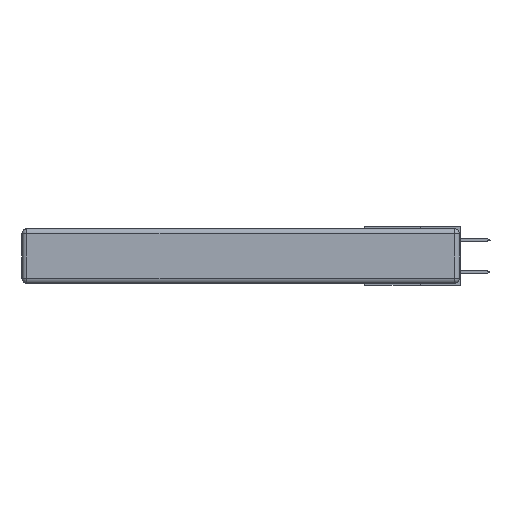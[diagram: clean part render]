
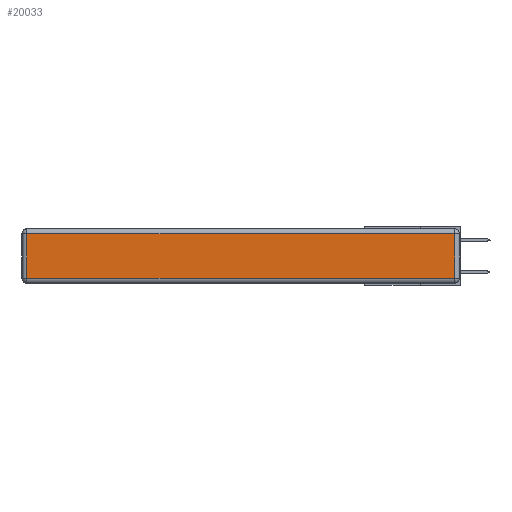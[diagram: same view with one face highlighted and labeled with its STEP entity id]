
A CAD part, left-side view. The second image highlights one B-rep face of the part: STEP entity #20033.
In plain terms, the highlighted planar face has unit normal (-1, 0, 0).
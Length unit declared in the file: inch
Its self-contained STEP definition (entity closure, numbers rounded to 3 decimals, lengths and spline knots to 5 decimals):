
#385 = DIRECTION ( 'NONE',  ( 0., 0., 1. ) ) ;
#3151 = DIRECTION ( 'NONE',  ( 0., 0., 1. ) ) ;
#3289 = VECTOR ( 'NONE', #29378, 39.37008 ) ;
#5413 = VECTOR ( 'NONE', #9314, 39.37008 ) ;
#5659 = VERTEX_POINT ( 'NONE', #28463 ) ;
#5773 = EDGE_CURVE ( 'NONE', #5659, #25443, #7020, .T. ) ;
#6443 = CARTESIAN_POINT ( 'NONE',  ( 0., 0.03, -0.313 ) ) ;
#6794 = VECTOR ( 'NONE', #29676, 39.37008 ) ;
#7020 = LINE ( 'NONE', #21925, #3289 ) ;
#9314 = DIRECTION ( 'NONE',  ( 0., -1., 0. ) ) ;
#10220 = EDGE_CURVE ( 'NONE', #22763, #5659, #13113, .T. ) ;
#11772 = LINE ( 'NONE', #13994, #5413 ) ;
#12462 = ORIENTED_EDGE ( 'NONE', *, *, #10220, .T. ) ;
#13113 = LINE ( 'NONE', #15194, #6794 ) ;
#13943 = CARTESIAN_POINT ( 'NONE',  ( 0., 0.03, -0.03 ) ) ;
#13994 = CARTESIAN_POINT ( 'NONE',  ( 0., 0., -0.313 ) ) ;
#14856 = ORIENTED_EDGE ( 'NONE', *, *, #5773, .T. ) ;
#15194 = CARTESIAN_POINT ( 'NONE',  ( 0., 2.75, -0.03 ) ) ;
#16718 = CARTESIAN_POINT ( 'NONE',  ( 0., 0.03, -0.343 ) ) ;
#17314 = AXIS2_PLACEMENT_3D ( 'NONE', #17500, #24898, #3151 ) ;
#17500 = CARTESIAN_POINT ( 'NONE',  ( 0., 0., -0.343 ) ) ;
#17806 = CARTESIAN_POINT ( 'NONE',  ( 0., 2.72, -0.313 ) ) ;
#19565 = EDGE_CURVE ( 'NONE', #25443, #20375, #11772, .T. ) ;
#20002 = PLANE ( 'NONE',  #17314 ) ;
#20033 = ADVANCED_FACE ( 'NONE', ( #21492 ), #20002, .T. ) ;
#20370 = ORIENTED_EDGE ( 'NONE', *, *, #19565, .T. ) ;
#20375 = VERTEX_POINT ( 'NONE', #6443 ) ;
#21114 = ORIENTED_EDGE ( 'NONE', *, *, #29300, .T. ) ;
#21492 = FACE_OUTER_BOUND ( 'NONE', #24614, .T. ) ;
#21925 = CARTESIAN_POINT ( 'NONE',  ( 0., 2.72, -0.343 ) ) ;
#22763 = VERTEX_POINT ( 'NONE', #13943 ) ;
#24614 = EDGE_LOOP ( 'NONE', ( #20370, #21114, #12462, #14856 ) ) ;
#24898 = DIRECTION ( 'NONE',  ( -1., 0., 0. ) ) ;
#25443 = VERTEX_POINT ( 'NONE', #17806 ) ;
#26232 = VECTOR ( 'NONE', #385, 39.37008 ) ;
#28463 = CARTESIAN_POINT ( 'NONE',  ( 0., 2.72, -0.03 ) ) ;
#29300 = EDGE_CURVE ( 'NONE', #20375, #22763, #29978, .T. ) ;
#29378 = DIRECTION ( 'NONE',  ( 0., 0., -1. ) ) ;
#29676 = DIRECTION ( 'NONE',  ( 0., 1., 0. ) ) ;
#29978 = LINE ( 'NONE', #16718, #26232 ) ;
